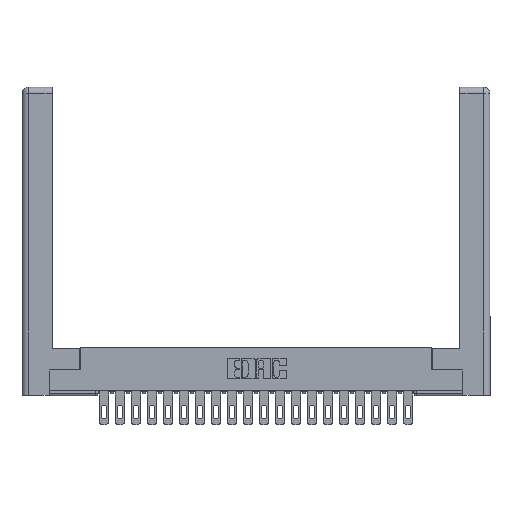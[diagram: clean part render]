
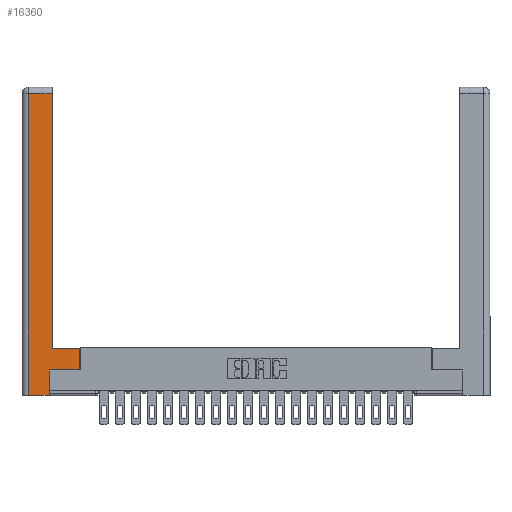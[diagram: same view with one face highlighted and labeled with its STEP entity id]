
A CAD part, top view. The second image highlights one B-rep face of the part: STEP entity #16360.
In plain terms, the highlighted planar face has unit normal (0, 0, 1).
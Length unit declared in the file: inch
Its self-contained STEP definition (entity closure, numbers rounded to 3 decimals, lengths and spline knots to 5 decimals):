
#244 = ORIENTED_EDGE ( 'NONE', *, *, #19010, .T. ) ;
#265 = LINE ( 'NONE', #5160, #15637 ) ;
#452 = FACE_OUTER_BOUND ( 'NONE', #13737, .T. ) ;
#674 = DIRECTION ( 'NONE',  ( 0., -1., 0. ) ) ;
#677 = EDGE_CURVE ( 'NONE', #6192, #13433, #21916, .T. ) ;
#1207 = CARTESIAN_POINT ( 'NONE',  ( 0.265, 0., 0. ) ) ;
#1963 = CARTESIAN_POINT ( 'NONE',  ( 0.0615, 2.94, 0. ) ) ;
#2137 = EDGE_CURVE ( 'NONE', #12643, #18073, #17701, .T. ) ;
#2195 = LINE ( 'NONE', #1963, #4174 ) ;
#2232 = CARTESIAN_POINT ( 'NONE',  ( 0.565, 0.245, 0. ) ) ;
#2275 = LINE ( 'NONE', #22325, #8238 ) ;
#2977 = VECTOR ( 'NONE', #16118, 39.37008 ) ;
#3218 = CARTESIAN_POINT ( 'NONE',  ( 0., 0., 0. ) ) ;
#3523 = CARTESIAN_POINT ( 'NONE',  ( 0.565, 0.245, 0. ) ) ;
#3632 = DIRECTION ( 'NONE',  ( 0., 0., -1. ) ) ;
#3782 = CARTESIAN_POINT ( 'NONE',  ( 0.265, 0.245, 0. ) ) ;
#3855 = PLANE ( 'NONE',  #9674 ) ;
#4079 = EDGE_CURVE ( 'NONE', #19102, #9448, #2195, .T. ) ;
#4105 = VERTEX_POINT ( 'NONE', #20961 ) ;
#4174 = VECTOR ( 'NONE', #15852, 39.37008 ) ;
#5160 = CARTESIAN_POINT ( 'NONE',  ( 0.565, 0.45, 0. ) ) ;
#5282 = VECTOR ( 'NONE', #5874, 39.37008 ) ;
#5874 = DIRECTION ( 'NONE',  ( -1., 0., 0. ) ) ;
#6192 = VERTEX_POINT ( 'NONE', #7747 ) ;
#6510 = ORIENTED_EDGE ( 'NONE', *, *, #677, .T. ) ;
#6814 = CARTESIAN_POINT ( 'NONE',  ( 0.0615, 2.94, 0. ) ) ;
#6912 = VECTOR ( 'NONE', #10723, 39.37008 ) ;
#7142 = EDGE_CURVE ( 'NONE', #22376, #4105, #8570, .T. ) ;
#7747 = CARTESIAN_POINT ( 'NONE',  ( 0.565, 0.45, 0. ) ) ;
#8238 = VECTOR ( 'NONE', #674, 39.37008 ) ;
#8570 = LINE ( 'NONE', #1207, #19554 ) ;
#9448 = VERTEX_POINT ( 'NONE', #6814 ) ;
#9674 = AXIS2_PLACEMENT_3D ( 'NONE', #3218, #3632, #18811 ) ;
#10723 = DIRECTION ( 'NONE',  ( 0., 1., 0. ) ) ;
#12564 = ORIENTED_EDGE ( 'NONE', *, *, #4079, .T. ) ;
#12626 = CARTESIAN_POINT ( 'NONE',  ( 0.295, 3., 0. ) ) ;
#12643 = VERTEX_POINT ( 'NONE', #12912 ) ;
#12912 = CARTESIAN_POINT ( 'NONE',  ( 0.265, 0.245, 0. ) ) ;
#12988 = ORIENTED_EDGE ( 'NONE', *, *, #7142, .T. ) ;
#13046 = CARTESIAN_POINT ( 'NONE',  ( 0.295, 0.45, 0. ) ) ;
#13433 = VERTEX_POINT ( 'NONE', #17870 ) ;
#13596 = DIRECTION ( 'NONE',  ( 1., 0., 0. ) ) ;
#13737 = EDGE_LOOP ( 'NONE', ( #244, #12564, #14971, #12988, #17431, #18912, #16345, #6510 ) ) ;
#14971 = ORIENTED_EDGE ( 'NONE', *, *, #16403, .T. ) ;
#15019 = CARTESIAN_POINT ( 'NONE',  ( 0.295, 2.94, 0. ) ) ;
#15637 = VECTOR ( 'NONE', #15969, 39.37008 ) ;
#15852 = DIRECTION ( 'NONE',  ( -1., 0., 0. ) ) ;
#15969 = DIRECTION ( 'NONE',  ( 0., 1., 0. ) ) ;
#16118 = DIRECTION ( 'NONE',  ( 1., 0., 0. ) ) ;
#16136 = CARTESIAN_POINT ( 'NONE',  ( 0.0615, 0., 0. ) ) ;
#16345 = ORIENTED_EDGE ( 'NONE', *, *, #21573, .T. ) ;
#16360 = ADVANCED_FACE ( 'NONE', ( #452 ), #3855, .F. ) ;
#16403 = EDGE_CURVE ( 'NONE', #9448, #22376, #2275, .T. ) ;
#16703 = VECTOR ( 'NONE', #19563, 39.37008 ) ;
#17431 = ORIENTED_EDGE ( 'NONE', *, *, #21626, .T. ) ;
#17701 = LINE ( 'NONE', #2232, #2977 ) ;
#17870 = CARTESIAN_POINT ( 'NONE',  ( 0.295, 0.45, 0. ) ) ;
#17975 = LINE ( 'NONE', #12626, #16703 ) ;
#18073 = VERTEX_POINT ( 'NONE', #3523 ) ;
#18811 = DIRECTION ( 'NONE',  ( -1., 0., 0. ) ) ;
#18912 = ORIENTED_EDGE ( 'NONE', *, *, #2137, .T. ) ;
#19010 = EDGE_CURVE ( 'NONE', #13433, #19102, #17975, .T. ) ;
#19102 = VERTEX_POINT ( 'NONE', #15019 ) ;
#19379 = LINE ( 'NONE', #3782, #6912 ) ;
#19554 = VECTOR ( 'NONE', #13596, 39.37008 ) ;
#19563 = DIRECTION ( 'NONE',  ( 0., 1., 0. ) ) ;
#20961 = CARTESIAN_POINT ( 'NONE',  ( 0.265, 0., 0. ) ) ;
#21573 = EDGE_CURVE ( 'NONE', #18073, #6192, #265, .T. ) ;
#21626 = EDGE_CURVE ( 'NONE', #4105, #12643, #19379, .T. ) ;
#21916 = LINE ( 'NONE', #13046, #5282 ) ;
#22325 = CARTESIAN_POINT ( 'NONE',  ( 0.0615, 0., 0. ) ) ;
#22376 = VERTEX_POINT ( 'NONE', #16136 ) ;
